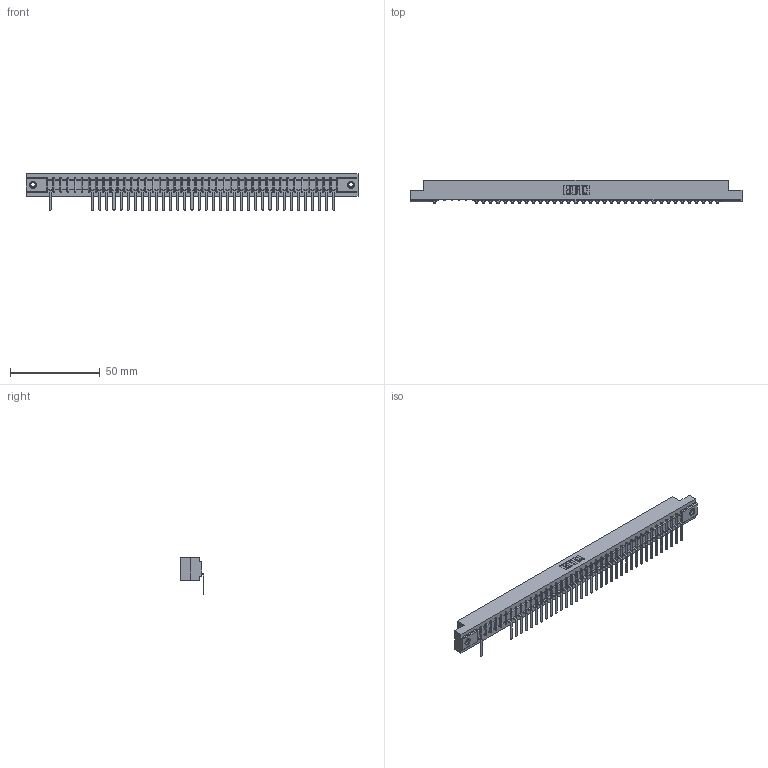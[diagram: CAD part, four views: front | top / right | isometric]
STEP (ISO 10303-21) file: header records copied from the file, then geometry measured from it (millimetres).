
FILE_DESCRIPTION (( 'STEP AP203' ), '1' );
FILE_NAME ('357-041-557-107.STEP', '2018-08-11T07:26:05', ( '' ), ( '' ), 'SwSTEP 2.0', 'SolidWorks 2016', '' );
FILE_SCHEMA (( 'CONFIG_CONTROL_DESIGN' ));
Length unit declared in the file: inch
Products named in the file (4): 345-250-001_345-250-005-103; 357-041-557-107; 307 Part_.156 Dia Mounting Holes; 307-290-002_557
Assembly tree (39 placements, depth 2):
  357-041-557-107
    307 Part_.156 Dia Mounting Holes
    307-290-002_557  x36
    345-250-001_345-250-005-103  x2
Bounding box: 185.47 x 13.32 x 20.66 mm (x, y, z)
Volume: 19779.2 mm3; surface area: 24584.8 mm2
Topology: 39 solids, 39 shells, 3128 faces, 9563 edges, 6254 vertices
Faces by surface type: plane 1854, cylinder 1174, sphere 84, cone 12, torus 4
Entity records: 37151 total; most frequent: CARTESIAN_POINT 6270, ORIENTED_EDGE 6258, DIRECTION 6097, EDGE_CURVE 3129, LINE 2395, VECTOR 2395, VERTEX_POINT 2024, AXIS2_PLACEMENT_3D 1851
